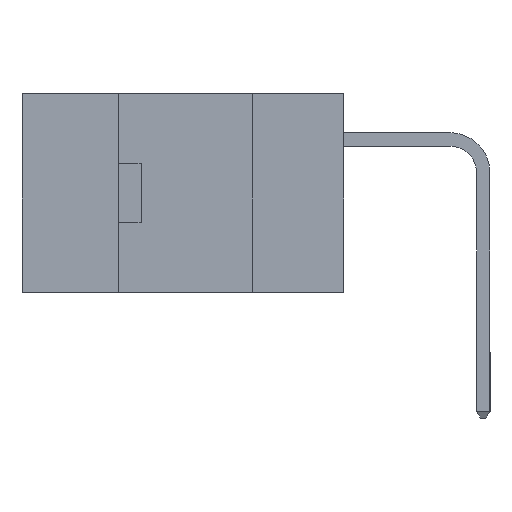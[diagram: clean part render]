
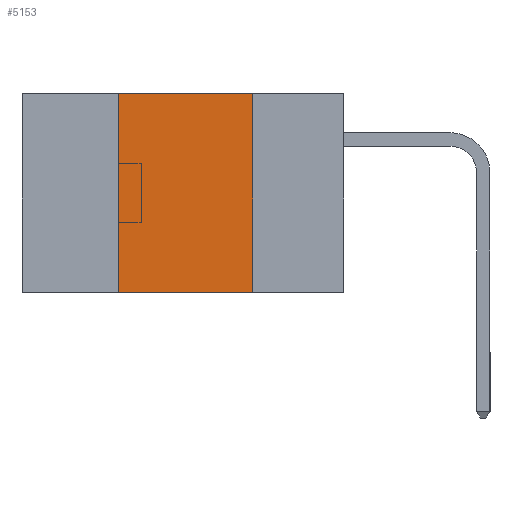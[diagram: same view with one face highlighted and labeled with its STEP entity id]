
A CAD part, left-side view. The second image highlights one B-rep face of the part: STEP entity #5153.
In plain terms, the highlighted planar face has unit normal (-1, 0, 0).
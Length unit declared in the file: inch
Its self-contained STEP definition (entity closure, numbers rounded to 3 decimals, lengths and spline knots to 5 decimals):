
#154 = ORIENTED_EDGE ( 'NONE', *, *, #13264, .F. ) ;
#1316 = LINE ( 'NONE', #5777, #17544 ) ;
#1604 = DIRECTION ( 'NONE',  ( 0., -1., 0. ) ) ;
#2013 = CARTESIAN_POINT ( 'NONE',  ( 0., 0.6, -0.37 ) ) ;
#2487 = CARTESIAN_POINT ( 'NONE',  ( 0., 0.42, -0.37 ) ) ;
#2934 = ORIENTED_EDGE ( 'NONE', *, *, #12875, .F. ) ;
#3295 = PLANE ( 'NONE',  #16101 ) ;
#4903 = DIRECTION ( 'NONE',  ( 0., 0., 1. ) ) ;
#5153 = ADVANCED_FACE ( 'NONE', ( #19725 ), #3295, .F. ) ;
#5539 = CARTESIAN_POINT ( 'NONE',  ( 0., 0.42, -0.37 ) ) ;
#5689 = ORIENTED_EDGE ( 'NONE', *, *, #13859, .F. ) ;
#5777 = CARTESIAN_POINT ( 'NONE',  ( 0., 0.17, -0.37 ) ) ;
#5913 = CARTESIAN_POINT ( 'NONE',  ( 0., 0.6, 0. ) ) ;
#6940 = DIRECTION ( 'NONE',  ( 0., 0., -1. ) ) ;
#7130 = VECTOR ( 'NONE', #1604, 39.37008 ) ;
#9617 = CARTESIAN_POINT ( 'NONE',  ( 0., 0.17, 0. ) ) ;
#10249 = ORIENTED_EDGE ( 'NONE', *, *, #23179, .T. ) ;
#10502 = CARTESIAN_POINT ( 'NONE',  ( 0., 0.42, 0. ) ) ;
#11965 = DIRECTION ( 'NONE',  ( 0., 0., -1. ) ) ;
#12875 = EDGE_CURVE ( 'NONE', #16019, #17149, #1316, .T. ) ;
#13128 = DIRECTION ( 'NONE',  ( 1., 0., 0. ) ) ;
#13264 = EDGE_CURVE ( 'NONE', #26299, #16019, #20172, .T. ) ;
#13859 = EDGE_CURVE ( 'NONE', #17910, #26299, #19441, .T. ) ;
#15292 = VECTOR ( 'NONE', #4903, 39.37008 ) ;
#16019 = VERTEX_POINT ( 'NONE', #9617 ) ;
#16101 = AXIS2_PLACEMENT_3D ( 'NONE', #17441, #13128, #6940 ) ;
#17149 = VERTEX_POINT ( 'NONE', #20282 ) ;
#17441 = CARTESIAN_POINT ( 'NONE',  ( 0., 0.6, 0. ) ) ;
#17544 = VECTOR ( 'NONE', #11965, 39.37008 ) ;
#17896 = DIRECTION ( 'NONE',  ( 0., -1., 0. ) ) ;
#17910 = VERTEX_POINT ( 'NONE', #5539 ) ;
#19441 = LINE ( 'NONE', #2487, #15292 ) ;
#19725 = FACE_OUTER_BOUND ( 'NONE', #23013, .T. ) ;
#20172 = LINE ( 'NONE', #5913, #26420 ) ;
#20282 = CARTESIAN_POINT ( 'NONE',  ( 0., 0.17, -0.37 ) ) ;
#20452 = LINE ( 'NONE', #2013, #7130 ) ;
#23013 = EDGE_LOOP ( 'NONE', ( #2934, #154, #5689, #10249 ) ) ;
#23179 = EDGE_CURVE ( 'NONE', #17910, #17149, #20452, .T. ) ;
#26299 = VERTEX_POINT ( 'NONE', #10502 ) ;
#26420 = VECTOR ( 'NONE', #17896, 39.37008 ) ;
